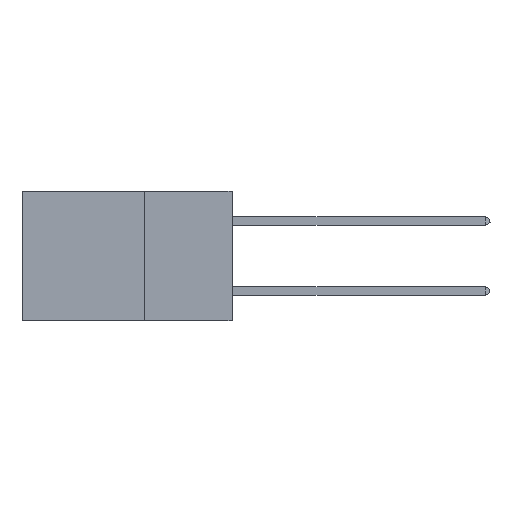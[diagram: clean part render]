
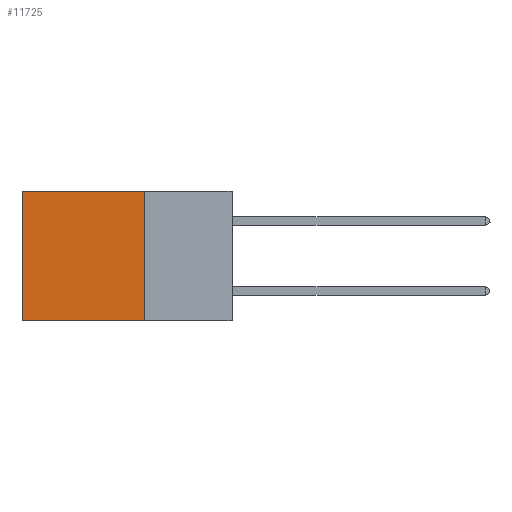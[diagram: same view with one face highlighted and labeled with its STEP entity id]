
A CAD part, left-side view. The second image highlights one B-rep face of the part: STEP entity #11725.
In plain terms, the highlighted planar face has unit normal (-1, 0, 0).
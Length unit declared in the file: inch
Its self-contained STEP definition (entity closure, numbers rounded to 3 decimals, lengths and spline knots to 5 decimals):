
#98 = EDGE_CURVE ( 'NONE', #21666, #13913, #13812, .T. ) ;
#844 = ORIENTED_EDGE ( 'NONE', *, *, #98, .F. ) ;
#1807 = EDGE_CURVE ( 'NONE', #20053, #15147, #15064, .T. ) ;
#1847 = AXIS2_PLACEMENT_3D ( 'NONE', #19568, #9616, #21183 ) ;
#3202 = EDGE_LOOP ( 'NONE', ( #20554, #17870, #844, #10267 ) ) ;
#3267 = CARTESIAN_POINT ( 'NONE',  ( 0.2875, 0.25, 0. ) ) ;
#4203 = DIRECTION ( 'NONE',  ( 0., 0., -1. ) ) ;
#4306 = CARTESIAN_POINT ( 'NONE',  ( 0.2875, 0.25, -0.37 ) ) ;
#5005 = DIRECTION ( 'NONE',  ( 0., 1., 0. ) ) ;
#5918 = CARTESIAN_POINT ( 'NONE',  ( 0.2875, 0.25, 0. ) ) ;
#7404 = LINE ( 'NONE', #4306, #11886 ) ;
#8222 = CARTESIAN_POINT ( 'NONE',  ( 0.2875, 0.6, 0. ) ) ;
#9371 = VECTOR ( 'NONE', #4203, 39.37008 ) ;
#9506 = CARTESIAN_POINT ( 'NONE',  ( 0.2875, 0.6, -0.37 ) ) ;
#9616 = DIRECTION ( 'NONE',  ( 1., 0., 0. ) ) ;
#10094 = VECTOR ( 'NONE', #5005, 39.37008 ) ;
#10267 = ORIENTED_EDGE ( 'NONE', *, *, #17965, .T. ) ;
#11725 = ADVANCED_FACE ( 'NONE', ( #12471 ), #16261, .F. ) ;
#11886 = VECTOR ( 'NONE', #16115, 39.37008 ) ;
#12471 = FACE_OUTER_BOUND ( 'NONE', #3202, .T. ) ;
#13812 = LINE ( 'NONE', #5918, #9371 ) ;
#13913 = VERTEX_POINT ( 'NONE', #21410 ) ;
#14000 = VECTOR ( 'NONE', #14993, 39.37008 ) ;
#14549 = LINE ( 'NONE', #3267, #10094 ) ;
#14907 = CARTESIAN_POINT ( 'NONE',  ( 0.2875, 0.6, 0. ) ) ;
#14993 = DIRECTION ( 'NONE',  ( 0., 0., -1. ) ) ;
#15064 = LINE ( 'NONE', #14907, #14000 ) ;
#15147 = VERTEX_POINT ( 'NONE', #9506 ) ;
#16094 = CARTESIAN_POINT ( 'NONE',  ( 0.2875, 0.25, 0. ) ) ;
#16115 = DIRECTION ( 'NONE',  ( 0., 1., 0. ) ) ;
#16261 = PLANE ( 'NONE',  #1847 ) ;
#17870 = ORIENTED_EDGE ( 'NONE', *, *, #19190, .F. ) ;
#17965 = EDGE_CURVE ( 'NONE', #21666, #20053, #14549, .T. ) ;
#19190 = EDGE_CURVE ( 'NONE', #13913, #15147, #7404, .T. ) ;
#19568 = CARTESIAN_POINT ( 'NONE',  ( 0.2875, 0.25, 0. ) ) ;
#20053 = VERTEX_POINT ( 'NONE', #8222 ) ;
#20554 = ORIENTED_EDGE ( 'NONE', *, *, #1807, .T. ) ;
#21183 = DIRECTION ( 'NONE',  ( 0., 0., -1. ) ) ;
#21410 = CARTESIAN_POINT ( 'NONE',  ( 0.2875, 0.25, -0.37 ) ) ;
#21666 = VERTEX_POINT ( 'NONE', #16094 ) ;
